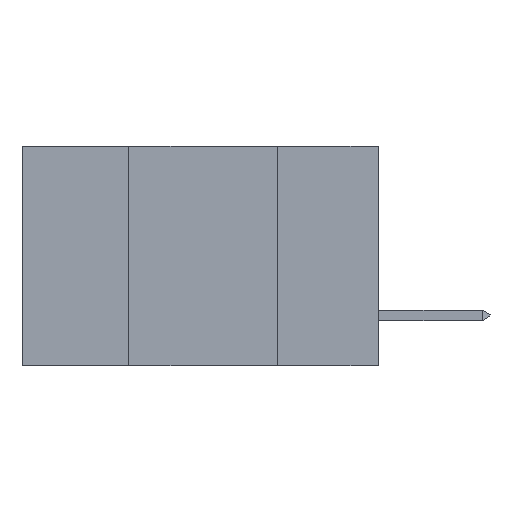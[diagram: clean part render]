
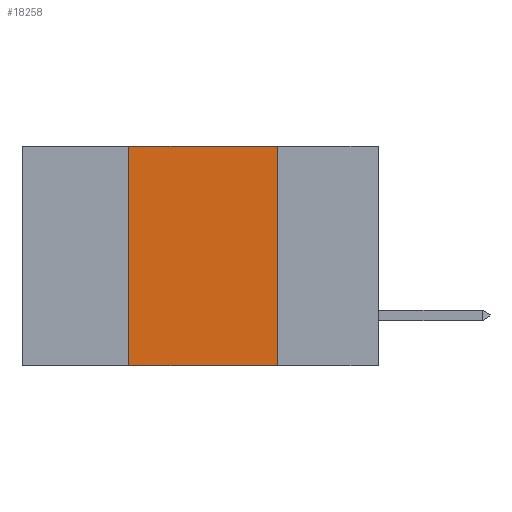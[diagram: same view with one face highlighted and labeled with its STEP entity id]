
A CAD part, left-side view. The second image highlights one B-rep face of the part: STEP entity #18258.
In plain terms, the highlighted planar face has unit normal (-1, 0, 0).
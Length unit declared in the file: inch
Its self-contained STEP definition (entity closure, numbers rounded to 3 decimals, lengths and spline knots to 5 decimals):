
#1234 = AXIS2_PLACEMENT_3D ( 'NONE', #8498, #5186, #20732 ) ;
#1235 = CARTESIAN_POINT ( 'NONE',  ( 0., 0.17, -0.37 ) ) ;
#1539 = VERTEX_POINT ( 'NONE', #1235 ) ;
#1700 = ORIENTED_EDGE ( 'NONE', *, *, #2349, .T. ) ;
#2349 = EDGE_CURVE ( 'NONE', #16035, #1539, #4917, .T. ) ;
#3002 = VECTOR ( 'NONE', #10542, 39.37008 ) ;
#3498 = VERTEX_POINT ( 'NONE', #3970 ) ;
#3970 = CARTESIAN_POINT ( 'NONE',  ( 0., 0.17, 0. ) ) ;
#4817 = DIRECTION ( 'NONE',  ( 0., 0., 1. ) ) ;
#4917 = LINE ( 'NONE', #6866, #3002 ) ;
#5186 = DIRECTION ( 'NONE',  ( 1., 0., 0. ) ) ;
#6866 = CARTESIAN_POINT ( 'NONE',  ( 0., 0.6, -0.37 ) ) ;
#7054 = VERTEX_POINT ( 'NONE', #9760 ) ;
#7183 = ORIENTED_EDGE ( 'NONE', *, *, #18340, .F. ) ;
#7287 = LINE ( 'NONE', #20764, #19127 ) ;
#8498 = CARTESIAN_POINT ( 'NONE',  ( 0., 0.6, 0. ) ) ;
#8577 = CARTESIAN_POINT ( 'NONE',  ( 0., 0.17, 0. ) ) ;
#9760 = CARTESIAN_POINT ( 'NONE',  ( 0., 0.42, 0. ) ) ;
#10191 = VECTOR ( 'NONE', #10791, 39.37008 ) ;
#10542 = DIRECTION ( 'NONE',  ( 0., -1., 0. ) ) ;
#10791 = DIRECTION ( 'NONE',  ( 0., -1., 0. ) ) ;
#13018 = FACE_OUTER_BOUND ( 'NONE', #17067, .T. ) ;
#13035 = ORIENTED_EDGE ( 'NONE', *, *, #17660, .F. ) ;
#16035 = VERTEX_POINT ( 'NONE', #21077 ) ;
#17067 = EDGE_LOOP ( 'NONE', ( #7183, #20046, #13035, #1700 ) ) ;
#17453 = LINE ( 'NONE', #8577, #21031 ) ;
#17660 = EDGE_CURVE ( 'NONE', #16035, #7054, #7287, .T. ) ;
#17792 = CARTESIAN_POINT ( 'NONE',  ( 0., 0.6, 0. ) ) ;
#18258 = ADVANCED_FACE ( 'NONE', ( #13018 ), #22486, .F. ) ;
#18340 = EDGE_CURVE ( 'NONE', #3498, #1539, #17453, .T. ) ;
#18889 = DIRECTION ( 'NONE',  ( 0., 0., -1. ) ) ;
#19127 = VECTOR ( 'NONE', #4817, 39.37008 ) ;
#20046 = ORIENTED_EDGE ( 'NONE', *, *, #21420, .F. ) ;
#20732 = DIRECTION ( 'NONE',  ( 0., 0., -1. ) ) ;
#20764 = CARTESIAN_POINT ( 'NONE',  ( 0., 0.42, 0. ) ) ;
#21031 = VECTOR ( 'NONE', #18889, 39.37008 ) ;
#21077 = CARTESIAN_POINT ( 'NONE',  ( 0., 0.42, -0.37 ) ) ;
#21420 = EDGE_CURVE ( 'NONE', #7054, #3498, #21731, .T. ) ;
#21731 = LINE ( 'NONE', #17792, #10191 ) ;
#22486 = PLANE ( 'NONE',  #1234 ) ;
